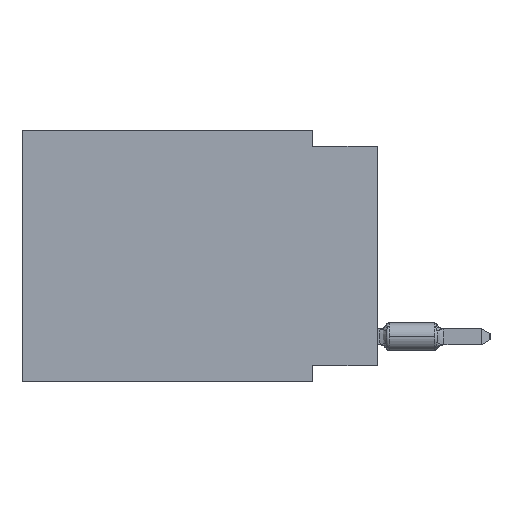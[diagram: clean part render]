
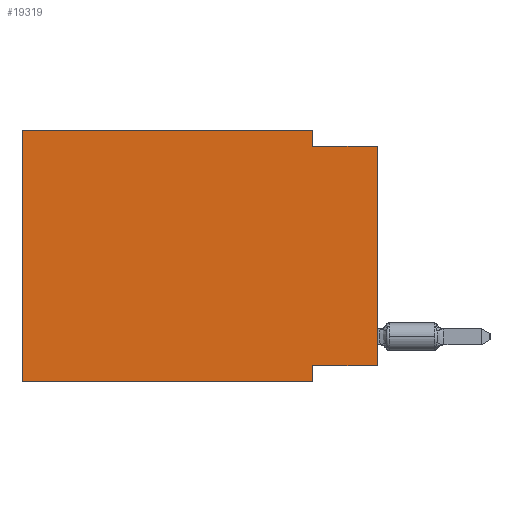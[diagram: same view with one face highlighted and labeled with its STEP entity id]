
A CAD part, left-side view. The second image highlights one B-rep face of the part: STEP entity #19319.
In plain terms, the highlighted planar face has unit normal (-1, 0, 0).
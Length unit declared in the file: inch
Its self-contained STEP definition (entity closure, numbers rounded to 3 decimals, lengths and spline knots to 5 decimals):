
#31 = VERTEX_POINT ( 'NONE', #136 ) ;
#76 = DIRECTION ( 'NONE',  ( 0., -1., 0. ) ) ;
#102 = CARTESIAN_POINT ( 'NONE',  ( 0., 0.55, 0. ) ) ;
#136 = CARTESIAN_POINT ( 'NONE',  ( 0., 0., -0.365 ) ) ;
#454 = DIRECTION ( 'NONE',  ( 0., 0., 1. ) ) ;
#562 = VECTOR ( 'NONE', #3398, 39.37008 ) ;
#751 = CARTESIAN_POINT ( 'NONE',  ( 0., 0., -0.365 ) ) ;
#1264 = LINE ( 'NONE', #20061, #4920 ) ;
#1808 = CARTESIAN_POINT ( 'NONE',  ( 0., 0.1, -0.025 ) ) ;
#3398 = DIRECTION ( 'NONE',  ( 0., -1., 0. ) ) ;
#3538 = CARTESIAN_POINT ( 'NONE',  ( 0., 0., -0.025 ) ) ;
#3972 = PLANE ( 'NONE',  #5980 ) ;
#4359 = VERTEX_POINT ( 'NONE', #3538 ) ;
#4374 = ORIENTED_EDGE ( 'NONE', *, *, #21780, .F. ) ;
#4920 = VECTOR ( 'NONE', #11897, 39.37008 ) ;
#5095 = CARTESIAN_POINT ( 'NONE',  ( 0., 0.55, -0.39 ) ) ;
#5441 = ORIENTED_EDGE ( 'NONE', *, *, #20518, .T. ) ;
#5635 = CARTESIAN_POINT ( 'NONE',  ( 0., 0.1, 0. ) ) ;
#5665 = VECTOR ( 'NONE', #19962, 39.37008 ) ;
#5980 = AXIS2_PLACEMENT_3D ( 'NONE', #102, #10629, #17337 ) ;
#6090 = VECTOR ( 'NONE', #6896, 39.37008 ) ;
#6548 = VERTEX_POINT ( 'NONE', #7825 ) ;
#6743 = EDGE_CURVE ( 'NONE', #20341, #6548, #15410, .T. ) ;
#6889 = DIRECTION ( 'NONE',  ( 0., 0., -1. ) ) ;
#6896 = DIRECTION ( 'NONE',  ( 0., 0., -1. ) ) ;
#7637 = DIRECTION ( 'NONE',  ( 0., 1., 0. ) ) ;
#7825 = CARTESIAN_POINT ( 'NONE',  ( 0., 0.1, -0.39 ) ) ;
#7834 = LINE ( 'NONE', #12940, #5665 ) ;
#8578 = EDGE_LOOP ( 'NONE', ( #16263, #15945, #16105, #13388, #4374, #5441, #12533, #19774 ) ) ;
#8580 = LINE ( 'NONE', #15971, #17211 ) ;
#10192 = LINE ( 'NONE', #5095, #562 ) ;
#10283 = VECTOR ( 'NONE', #76, 39.37008 ) ;
#10629 = DIRECTION ( 'NONE',  ( 1., 0., 0. ) ) ;
#10765 = VECTOR ( 'NONE', #7637, 39.37008 ) ;
#11897 = DIRECTION ( 'NONE',  ( 0., 0., 1. ) ) ;
#12533 = ORIENTED_EDGE ( 'NONE', *, *, #6743, .F. ) ;
#12669 = EDGE_CURVE ( 'NONE', #12754, #22322, #20610, .T. ) ;
#12754 = VERTEX_POINT ( 'NONE', #5635 ) ;
#12940 = CARTESIAN_POINT ( 'NONE',  ( 0., 0.55, 0. ) ) ;
#13388 = ORIENTED_EDGE ( 'NONE', *, *, #14378, .F. ) ;
#14255 = FACE_OUTER_BOUND ( 'NONE', #8578, .T. ) ;
#14378 = EDGE_CURVE ( 'NONE', #14798, #12754, #7834, .T. ) ;
#14798 = VERTEX_POINT ( 'NONE', #16721 ) ;
#15099 = EDGE_CURVE ( 'NONE', #31, #20341, #16262, .T. ) ;
#15410 = LINE ( 'NONE', #15528, #6090 ) ;
#15528 = CARTESIAN_POINT ( 'NONE',  ( 0., 0.1, -0.39 ) ) ;
#15945 = ORIENTED_EDGE ( 'NONE', *, *, #18001, .F. ) ;
#15971 = CARTESIAN_POINT ( 'NONE',  ( 0., 0., 0. ) ) ;
#16105 = ORIENTED_EDGE ( 'NONE', *, *, #12669, .F. ) ;
#16262 = LINE ( 'NONE', #751, #10765 ) ;
#16263 = ORIENTED_EDGE ( 'NONE', *, *, #20841, .T. ) ;
#16721 = CARTESIAN_POINT ( 'NONE',  ( 0., 0.55, 0. ) ) ;
#17211 = VECTOR ( 'NONE', #454, 39.37008 ) ;
#17337 = DIRECTION ( 'NONE',  ( 0., 0., -1. ) ) ;
#17465 = CARTESIAN_POINT ( 'NONE',  ( 0., 0.55, -0.39 ) ) ;
#18001 = EDGE_CURVE ( 'NONE', #22322, #4359, #20795, .T. ) ;
#18905 = CARTESIAN_POINT ( 'NONE',  ( 0., 0.1, 0. ) ) ;
#19319 = ADVANCED_FACE ( 'NONE', ( #14255 ), #3972, .F. ) ;
#19373 = VECTOR ( 'NONE', #6889, 39.37008 ) ;
#19774 = ORIENTED_EDGE ( 'NONE', *, *, #15099, .F. ) ;
#19962 = DIRECTION ( 'NONE',  ( 0., -1., 0. ) ) ;
#20061 = CARTESIAN_POINT ( 'NONE',  ( 0., 0.55, 0. ) ) ;
#20181 = VERTEX_POINT ( 'NONE', #17465 ) ;
#20182 = CARTESIAN_POINT ( 'NONE',  ( 0., 0.1, -0.365 ) ) ;
#20341 = VERTEX_POINT ( 'NONE', #20182 ) ;
#20518 = EDGE_CURVE ( 'NONE', #20181, #6548, #10192, .T. ) ;
#20610 = LINE ( 'NONE', #18905, #19373 ) ;
#20795 = LINE ( 'NONE', #20911, #10283 ) ;
#20841 = EDGE_CURVE ( 'NONE', #31, #4359, #8580, .T. ) ;
#20911 = CARTESIAN_POINT ( 'NONE',  ( 0., 0., -0.025 ) ) ;
#21780 = EDGE_CURVE ( 'NONE', #20181, #14798, #1264, .T. ) ;
#22322 = VERTEX_POINT ( 'NONE', #1808 ) ;
